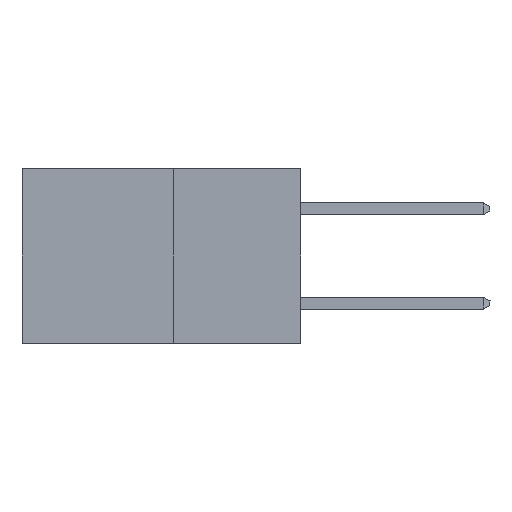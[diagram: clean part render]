
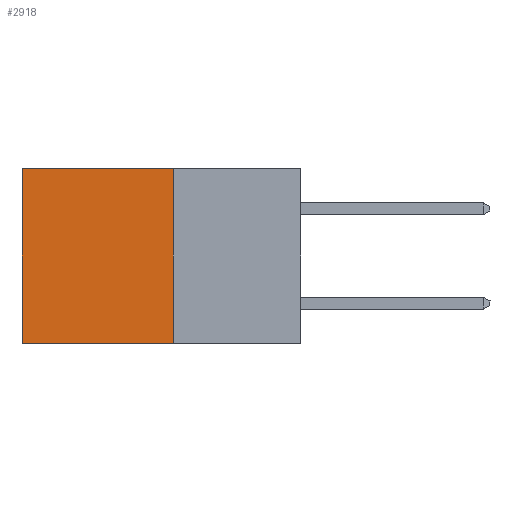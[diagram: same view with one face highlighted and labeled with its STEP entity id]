
A CAD part, left-side view. The second image highlights one B-rep face of the part: STEP entity #2918.
In plain terms, the highlighted planar face has unit normal (-1, 0, 0).
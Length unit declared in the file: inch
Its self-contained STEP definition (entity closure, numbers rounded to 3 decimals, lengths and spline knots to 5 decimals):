
#16 = ORIENTED_EDGE ( 'NONE', *, *, #8298, .F. ) ;
#66 = CARTESIAN_POINT ( 'NONE',  ( 0.277, 0.27, -0.37 ) ) ;
#293 = VERTEX_POINT ( 'NONE', #6437 ) ;
#407 = LINE ( 'NONE', #5962, #4519 ) ;
#1572 = EDGE_LOOP ( 'NONE', ( #3052, #7438, #16, #4381 ) ) ;
#1577 = VECTOR ( 'NONE', #4585, 39.37008 ) ;
#2055 = CARTESIAN_POINT ( 'NONE',  ( 0.277, 0.27, 0. ) ) ;
#2230 = EDGE_CURVE ( 'NONE', #293, #8138, #4817, .T. ) ;
#2918 = ADVANCED_FACE ( 'NONE', ( #6041 ), #6218, .F. ) ;
#2983 = CARTESIAN_POINT ( 'NONE',  ( 0.277, 0.27, 0. ) ) ;
#3052 = ORIENTED_EDGE ( 'NONE', *, *, #8427, .T. ) ;
#4009 = EDGE_CURVE ( 'NONE', #9485, #9533, #8625, .T. ) ;
#4381 = ORIENTED_EDGE ( 'NONE', *, *, #4009, .T. ) ;
#4519 = VECTOR ( 'NONE', #7556, 39.37008 ) ;
#4585 = DIRECTION ( 'NONE',  ( 0., 0., -1. ) ) ;
#4626 = AXIS2_PLACEMENT_3D ( 'NONE', #66, #10096, #10282 ) ;
#4817 = LINE ( 'NONE', #9397, #6967 ) ;
#4863 = DIRECTION ( 'NONE',  ( 0., 1., 0. ) ) ;
#5962 = CARTESIAN_POINT ( 'NONE',  ( 0.277, 0.27, -0.37 ) ) ;
#6041 = FACE_OUTER_BOUND ( 'NONE', #1572, .T. ) ;
#6218 = PLANE ( 'NONE',  #4626 ) ;
#6238 = CARTESIAN_POINT ( 'NONE',  ( 0.277, 0.59, -0.37 ) ) ;
#6437 = CARTESIAN_POINT ( 'NONE',  ( 0.277, 0.27, -0.37 ) ) ;
#6967 = VECTOR ( 'NONE', #4863, 39.37008 ) ;
#7438 = ORIENTED_EDGE ( 'NONE', *, *, #2230, .F. ) ;
#7556 = DIRECTION ( 'NONE',  ( 0., 0., -1. ) ) ;
#7815 = LINE ( 'NONE', #6238, #1577 ) ;
#7937 = CARTESIAN_POINT ( 'NONE',  ( 0.277, 0.59, 0. ) ) ;
#8138 = VERTEX_POINT ( 'NONE', #8935 ) ;
#8298 = EDGE_CURVE ( 'NONE', #9485, #293, #407, .T. ) ;
#8427 = EDGE_CURVE ( 'NONE', #9533, #8138, #7815, .T. ) ;
#8625 = LINE ( 'NONE', #2055, #10252 ) ;
#8935 = CARTESIAN_POINT ( 'NONE',  ( 0.277, 0.59, -0.37 ) ) ;
#9397 = CARTESIAN_POINT ( 'NONE',  ( 0.277, 0.27, -0.37 ) ) ;
#9485 = VERTEX_POINT ( 'NONE', #2983 ) ;
#9533 = VERTEX_POINT ( 'NONE', #7937 ) ;
#10081 = DIRECTION ( 'NONE',  ( 0., 1., 0. ) ) ;
#10096 = DIRECTION ( 'NONE',  ( 1., 0., 0. ) ) ;
#10252 = VECTOR ( 'NONE', #10081, 39.37008 ) ;
#10282 = DIRECTION ( 'NONE',  ( 0., 0., -1. ) ) ;
